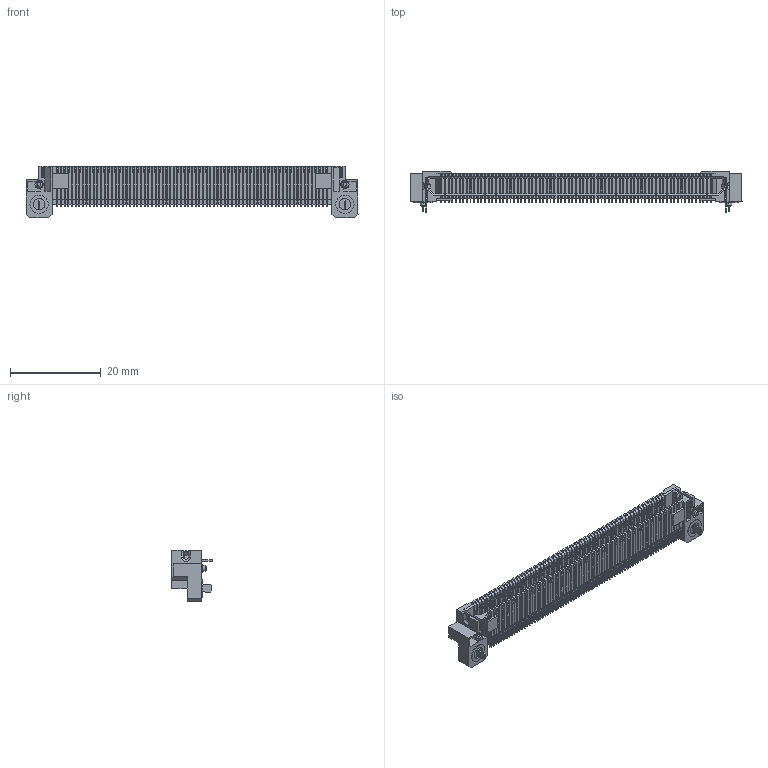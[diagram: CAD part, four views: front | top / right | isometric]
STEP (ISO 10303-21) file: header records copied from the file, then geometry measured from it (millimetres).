
FILE_DESCRIPTION (( 'STEP AP214' ), '1' );
FILE_NAME ('473-150-571-102.STEP', '2020-05-21T13:20:07', ( '' ), ( '' ), 'SwSTEP 2.0', 'SolidWorks 2020', '' );
FILE_SCHEMA (( 'AUTOMOTIVE_DESIGN' ));
Length unit declared in the file: millimetre
Products named in the file (7): 473-150-571-002 INS; 473 Contacts; 473 Latch LH; 473-150-571-102; 473 Contacts_Short; 473 Latch RH; 473 BM
Assembly tree (80 placements, depth 2):
  473-150-571-102
    473-150-571-002 INS
    473 BM  x2
    473 Contacts_Short  x2
    473 Contacts  x73
    473 Latch LH
    473 Latch RH
Bounding box: 73 x 9.02 x 11.35 mm (x, y, z)
Volume: 2021.7 mm3; surface area: 9903.1 mm2
Topology: 155 solids, 155 shells, 6295 faces, 17710 edges, 11732 vertices
Faces by surface type: plane 5134, cylinder 1154, cone 7
Entity records: 99156 total; most frequent: CARTESIAN_POINT 17688, ORIENTED_EDGE 17556, DIRECTION 15958, EDGE_CURVE 8778, LINE 7790, VECTOR 7790, VERTEX_POINT 5778, AXIS2_PLACEMENT_3D 4084
